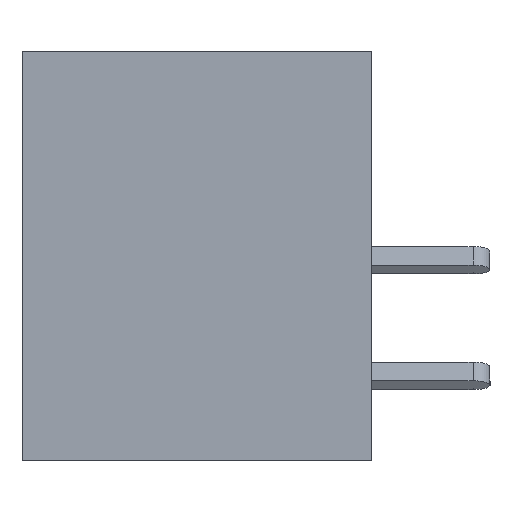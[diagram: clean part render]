
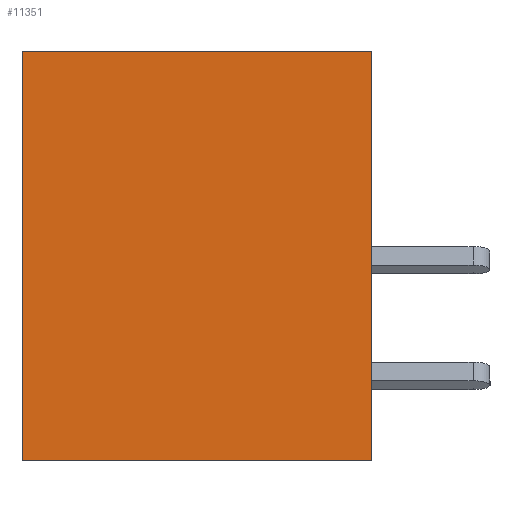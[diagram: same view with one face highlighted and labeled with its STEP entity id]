
A CAD part, left-side view. The second image highlights one B-rep face of the part: STEP entity #11351.
In plain terms, the highlighted planar face has unit normal (-1, 0, 0).
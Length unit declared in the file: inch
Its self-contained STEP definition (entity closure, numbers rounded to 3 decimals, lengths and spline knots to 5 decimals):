
#203 = CARTESIAN_POINT ( 'NONE',  ( 0., 0.453, 0. ) ) ;
#677 = LINE ( 'NONE', #16448, #5027 ) ;
#718 = DIRECTION ( 'NONE',  ( 0., -1., 0. ) ) ;
#1273 = LINE ( 'NONE', #15194, #16503 ) ;
#1303 = CARTESIAN_POINT ( 'NONE',  ( 0., 0., 0. ) ) ;
#1460 = PLANE ( 'NONE',  #10447 ) ;
#2044 = DIRECTION ( 'NONE',  ( 0., 0., 1. ) ) ;
#2856 = VERTEX_POINT ( 'NONE', #16103 ) ;
#4391 = EDGE_CURVE ( 'NONE', #2856, #5292, #1273, .T. ) ;
#4453 = CARTESIAN_POINT ( 'NONE',  ( 0., 0.453, -0.531 ) ) ;
#4846 = EDGE_LOOP ( 'NONE', ( #11744, #14695, #9413, #12006 ) ) ;
#5027 = VECTOR ( 'NONE', #2044, 39.37008 ) ;
#5292 = VERTEX_POINT ( 'NONE', #1303 ) ;
#5834 = DIRECTION ( 'NONE',  ( 0., -1., 0. ) ) ;
#6743 = LINE ( 'NONE', #203, #12492 ) ;
#7194 = EDGE_CURVE ( 'NONE', #11069, #2856, #6743, .T. ) ;
#7916 = DIRECTION ( 'NONE',  ( 0., 0., -1. ) ) ;
#8171 = EDGE_CURVE ( 'NONE', #11069, #14504, #12046, .T. ) ;
#9413 = ORIENTED_EDGE ( 'NONE', *, *, #7194, .F. ) ;
#9423 = DIRECTION ( 'NONE',  ( 0., 0., 1. ) ) ;
#9684 = EDGE_CURVE ( 'NONE', #14504, #5292, #677, .T. ) ;
#9897 = CARTESIAN_POINT ( 'NONE',  ( 0., 0.453, -0.531 ) ) ;
#10447 = AXIS2_PLACEMENT_3D ( 'NONE', #14469, #13121, #7916 ) ;
#10500 = CARTESIAN_POINT ( 'NONE',  ( 0., 0., -0.531 ) ) ;
#10956 = FACE_OUTER_BOUND ( 'NONE', #4846, .T. ) ;
#11069 = VERTEX_POINT ( 'NONE', #9897 ) ;
#11351 = ADVANCED_FACE ( 'NONE', ( #10956 ), #1460, .F. ) ;
#11744 = ORIENTED_EDGE ( 'NONE', *, *, #9684, .T. ) ;
#12006 = ORIENTED_EDGE ( 'NONE', *, *, #8171, .T. ) ;
#12046 = LINE ( 'NONE', #4453, #13690 ) ;
#12492 = VECTOR ( 'NONE', #9423, 39.37008 ) ;
#13121 = DIRECTION ( 'NONE',  ( 1., 0., 0. ) ) ;
#13690 = VECTOR ( 'NONE', #5834, 39.37008 ) ;
#14469 = CARTESIAN_POINT ( 'NONE',  ( 0., 0.453, 0. ) ) ;
#14504 = VERTEX_POINT ( 'NONE', #10500 ) ;
#14695 = ORIENTED_EDGE ( 'NONE', *, *, #4391, .F. ) ;
#15194 = CARTESIAN_POINT ( 'NONE',  ( 0., 0.453, 0. ) ) ;
#16103 = CARTESIAN_POINT ( 'NONE',  ( 0., 0.453, 0. ) ) ;
#16448 = CARTESIAN_POINT ( 'NONE',  ( 0., 0., 0. ) ) ;
#16503 = VECTOR ( 'NONE', #718, 39.37008 ) ;
